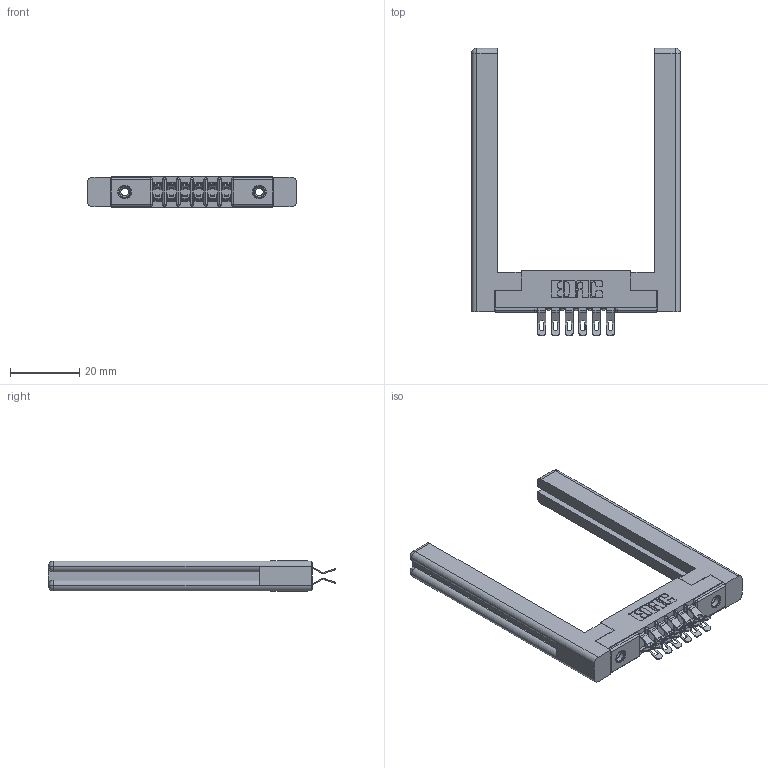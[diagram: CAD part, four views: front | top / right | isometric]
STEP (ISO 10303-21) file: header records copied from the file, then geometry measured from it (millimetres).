
FILE_DESCRIPTION (( 'STEP AP203' ), '1' );
FILE_NAME ('357-012-555-258.STEP', '2019-09-17T18:05:39', ( '' ), ( '' ), 'SwSTEP 2.0', 'SolidWorks 2016', '' );
FILE_SCHEMA (( 'CONFIG_CONTROL_DESIGN' ));
Length unit declared in the file: inch
Products named in the file (5): 307-220-058; 307 Part_.156 Dia Mounting Holes; 307-290-001_555; 345-250-001_345-250-001-102; 357-012-555-258
Assembly tree (17 placements, depth 2):
  357-012-555-258
    307 Part_.156 Dia Mounting Holes
    307-290-001_555  x12
    307-220-058  x2
    345-250-001_345-250-001-102  x2
Bounding box: 60.4 x 83.06 x 8.71 mm (x, y, z)
Volume: 11675 mm3; surface area: 11497.1 mm2
Topology: 17 solids, 17 shells, 999 faces, 2849 edges, 1850 vertices
Faces by surface type: plane 562, cylinder 399, sphere 14, torus 12, cone 12
Entity records: 12944 total; most frequent: CARTESIAN_POINT 2153, DIRECTION 2089, ORIENTED_EDGE 2074, EDGE_CURVE 1037, VECTOR 765, LINE 765, VERTEX_POINT 672, AXIS2_PLACEMENT_3D 662
